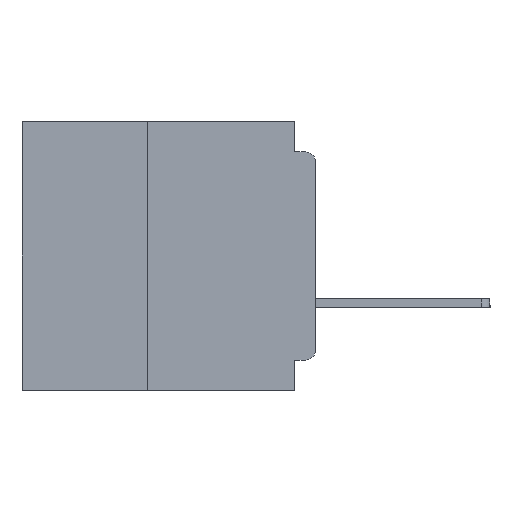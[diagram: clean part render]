
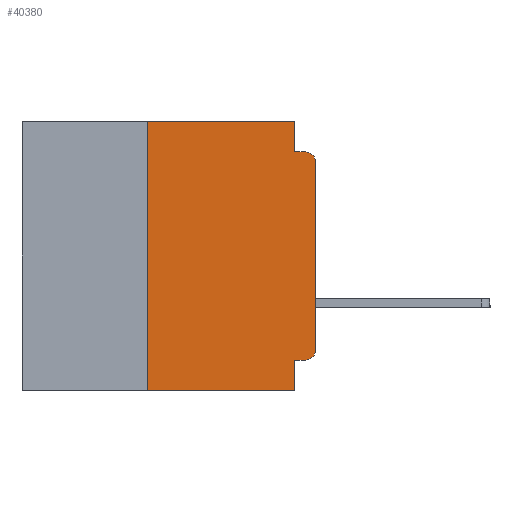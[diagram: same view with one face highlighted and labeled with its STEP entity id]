
A CAD part, left-side view. The second image highlights one B-rep face of the part: STEP entity #40380.
In plain terms, the highlighted planar face has unit normal (-1, 0, 0).
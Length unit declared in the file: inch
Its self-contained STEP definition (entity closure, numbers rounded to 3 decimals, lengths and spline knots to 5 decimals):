
#1002 = LINE ( 'NONE', #1820, #18404 ) ;
#1289 = EDGE_CURVE ( 'NONE', #6744, #9455, #9769, .T. ) ;
#1536 = DIRECTION ( 'NONE',  ( -1., 0., 0. ) ) ;
#1820 = CARTESIAN_POINT ( 'NONE',  ( 0., 0., -0.045 ) ) ;
#1826 = VERTEX_POINT ( 'NONE', #23283 ) ;
#2171 = DIRECTION ( 'NONE',  ( 0., 0., -1. ) ) ;
#3314 = EDGE_CURVE ( 'NONE', #24428, #22783, #46043, .T. ) ;
#3612 = ORIENTED_EDGE ( 'NONE', *, *, #44070, .T. ) ;
#3671 = DIRECTION ( 'NONE',  ( 0., 0., -1. ) ) ;
#3722 = CARTESIAN_POINT ( 'NONE',  ( 0., 0.031, 0. ) ) ;
#4293 = FACE_OUTER_BOUND ( 'NONE', #25309, .T. ) ;
#5847 = EDGE_CURVE ( 'NONE', #43277, #36932, #38964, .T. ) ;
#6160 = LINE ( 'NONE', #15997, #14865 ) ;
#6744 = VERTEX_POINT ( 'NONE', #3722 ) ;
#7448 = VERTEX_POINT ( 'NONE', #26020 ) ;
#8048 = DIRECTION ( 'NONE',  ( 0., 0., 1. ) ) ;
#8327 = CARTESIAN_POINT ( 'NONE',  ( 0., 0., 0. ) ) ;
#9380 = CARTESIAN_POINT ( 'NONE',  ( 0., 0.031, -0.355 ) ) ;
#9455 = VERTEX_POINT ( 'NONE', #37630 ) ;
#9729 = VECTOR ( 'NONE', #8048, 39.37008 ) ;
#9769 = LINE ( 'NONE', #40521, #17213 ) ;
#10287 = DIRECTION ( 'NONE',  ( 0., 0., -1. ) ) ;
#11048 = DIRECTION ( 'NONE',  ( 0., 0., 1. ) ) ;
#11424 = LINE ( 'NONE', #12774, #39469 ) ;
#12774 = CARTESIAN_POINT ( 'NONE',  ( 0., 0.437, -0.4 ) ) ;
#14395 = CARTESIAN_POINT ( 'NONE',  ( 0., 0.031, -0.4 ) ) ;
#14519 = VECTOR ( 'NONE', #27649, 39.37008 ) ;
#14865 = VECTOR ( 'NONE', #41616, 39.37008 ) ;
#15112 = VERTEX_POINT ( 'NONE', #43196 ) ;
#15997 = CARTESIAN_POINT ( 'NONE',  ( 0., 0., -0.355 ) ) ;
#16311 = CIRCLE ( 'NONE', #45704, 0.015 ) ;
#16445 = DIRECTION ( 'NONE',  ( 0., -1., 0. ) ) ;
#16449 = CARTESIAN_POINT ( 'NONE',  ( 0., 0., -0.34 ) ) ;
#17213 = VECTOR ( 'NONE', #10287, 39.37008 ) ;
#17731 = VERTEX_POINT ( 'NONE', #24430 ) ;
#18385 = EDGE_CURVE ( 'NONE', #17731, #43277, #39715, .T. ) ;
#18396 = ORIENTED_EDGE ( 'NONE', *, *, #31105, .F. ) ;
#18404 = VECTOR ( 'NONE', #27559, 39.37008 ) ;
#19006 = DIRECTION ( 'NONE',  ( 0., -1., 0. ) ) ;
#20436 = LINE ( 'NONE', #41038, #21594 ) ;
#21594 = VECTOR ( 'NONE', #19006, 39.37008 ) ;
#21606 = ORIENTED_EDGE ( 'NONE', *, *, #5847, .T. ) ;
#22016 = PLANE ( 'NONE',  #43689 ) ;
#22217 = VECTOR ( 'NONE', #11048, 39.37008 ) ;
#22783 = VERTEX_POINT ( 'NONE', #14395 ) ;
#23283 = CARTESIAN_POINT ( 'NONE',  ( 0., 0.015, -0.045 ) ) ;
#23597 = CARTESIAN_POINT ( 'NONE',  ( 0., 0.015, -0.06 ) ) ;
#24073 = EDGE_CURVE ( 'NONE', #15112, #7448, #31942, .T. ) ;
#24080 = ORIENTED_EDGE ( 'NONE', *, *, #27256, .T. ) ;
#24215 = DIRECTION ( 'NONE',  ( -1., 0., 0. ) ) ;
#24428 = VERTEX_POINT ( 'NONE', #9380 ) ;
#24430 = CARTESIAN_POINT ( 'NONE',  ( 0., 0.015, -0.355 ) ) ;
#25309 = EDGE_LOOP ( 'NONE', ( #21606, #3612, #18396, #37312, #33475, #42375, #24080, #30584, #33621, #34294 ) ) ;
#25456 = EDGE_CURVE ( 'NONE', #7448, #6744, #20436, .T. ) ;
#25651 = DIRECTION ( 'NONE',  ( 1., 0., 0. ) ) ;
#26020 = CARTESIAN_POINT ( 'NONE',  ( 0., 0.25, 0. ) ) ;
#26273 = AXIS2_PLACEMENT_3D ( 'NONE', #46296, #24215, #2171 ) ;
#27183 = EDGE_CURVE ( 'NONE', #17731, #24428, #6160, .T. ) ;
#27256 = EDGE_CURVE ( 'NONE', #15112, #22783, #11424, .T. ) ;
#27291 = DIRECTION ( 'NONE',  ( 0., 0., -1. ) ) ;
#27559 = DIRECTION ( 'NONE',  ( 0., -1., 0. ) ) ;
#27649 = DIRECTION ( 'NONE',  ( 0., 0., -1. ) ) ;
#30584 = ORIENTED_EDGE ( 'NONE', *, *, #3314, .F. ) ;
#31105 = EDGE_CURVE ( 'NONE', #9455, #1826, #1002, .T. ) ;
#31942 = LINE ( 'NONE', #32868, #22217 ) ;
#32020 = CARTESIAN_POINT ( 'NONE',  ( 0., 0., -0.06 ) ) ;
#32598 = CARTESIAN_POINT ( 'NONE',  ( 0., 0.031, -0.4 ) ) ;
#32868 = CARTESIAN_POINT ( 'NONE',  ( 0., 0.25, -0.4 ) ) ;
#33475 = ORIENTED_EDGE ( 'NONE', *, *, #25456, .F. ) ;
#33621 = ORIENTED_EDGE ( 'NONE', *, *, #27183, .F. ) ;
#34294 = ORIENTED_EDGE ( 'NONE', *, *, #18385, .T. ) ;
#36932 = VERTEX_POINT ( 'NONE', #32020 ) ;
#37312 = ORIENTED_EDGE ( 'NONE', *, *, #1289, .F. ) ;
#37630 = CARTESIAN_POINT ( 'NONE',  ( 0., 0.031, -0.045 ) ) ;
#38964 = LINE ( 'NONE', #8327, #9729 ) ;
#39469 = VECTOR ( 'NONE', #16445, 39.37008 ) ;
#39715 = CIRCLE ( 'NONE', #26273, 0.015 ) ;
#40380 = ADVANCED_FACE ( 'NONE', ( #4293 ), #22016, .F. ) ;
#40521 = CARTESIAN_POINT ( 'NONE',  ( 0., 0.031, 0. ) ) ;
#41038 = CARTESIAN_POINT ( 'NONE',  ( 0., 0.437, 0. ) ) ;
#41616 = DIRECTION ( 'NONE',  ( 0., 1., 0. ) ) ;
#42375 = ORIENTED_EDGE ( 'NONE', *, *, #24073, .F. ) ;
#43196 = CARTESIAN_POINT ( 'NONE',  ( 0., 0.25, -0.4 ) ) ;
#43277 = VERTEX_POINT ( 'NONE', #16449 ) ;
#43689 = AXIS2_PLACEMENT_3D ( 'NONE', #47734, #25651, #3671 ) ;
#44070 = EDGE_CURVE ( 'NONE', #36932, #1826, #16311, .T. ) ;
#45704 = AXIS2_PLACEMENT_3D ( 'NONE', #23597, #1536, #27291 ) ;
#46043 = LINE ( 'NONE', #32598, #14519 ) ;
#46296 = CARTESIAN_POINT ( 'NONE',  ( 0., 0.015, -0.34 ) ) ;
#47734 = CARTESIAN_POINT ( 'NONE',  ( 0., 0.437, 0. ) ) ;
